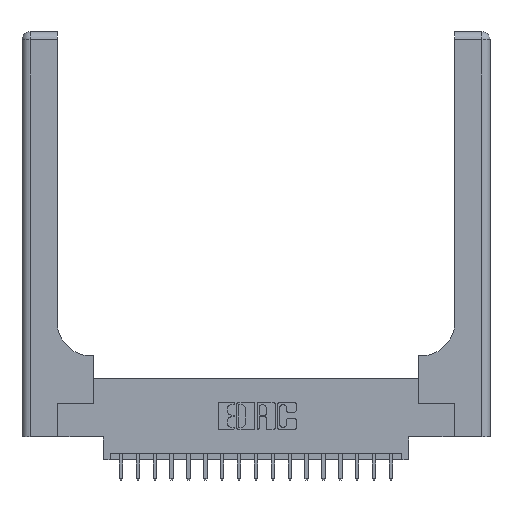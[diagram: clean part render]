
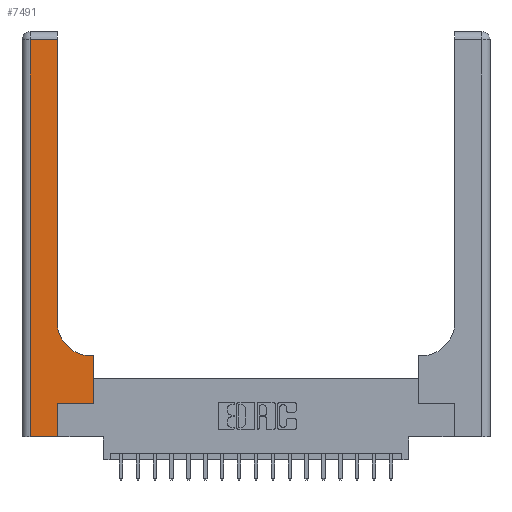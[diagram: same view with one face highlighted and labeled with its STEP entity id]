
A CAD part, top view. The second image highlights one B-rep face of the part: STEP entity #7491.
In plain terms, the highlighted planar face has unit normal (0, 0, 1).
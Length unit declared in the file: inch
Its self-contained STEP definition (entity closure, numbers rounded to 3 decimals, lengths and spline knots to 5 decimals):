
#865 = ORIENTED_EDGE ( 'NONE', *, *, #10429, .T. ) ;
#1348 = EDGE_CURVE ( 'NONE', #14793, #5308, #19549, .T. ) ;
#1537 = CARTESIAN_POINT ( 'NONE',  ( 0.265, 0.25, 0.37 ) ) ;
#1739 = VECTOR ( 'NONE', #1818, 39.37008 ) ;
#1818 = DIRECTION ( 'NONE',  ( 0., -1., 0. ) ) ;
#1980 = DIRECTION ( 'NONE',  ( 0., 1., 0. ) ) ;
#2242 = LINE ( 'NONE', #11277, #1739 ) ;
#2563 = CIRCLE ( 'NONE', #2577, 0.25 ) ;
#2577 = AXIS2_PLACEMENT_3D ( 'NONE', #15284, #6042, #16761 ) ;
#2864 = VERTEX_POINT ( 'NONE', #17548 ) ;
#2959 = CARTESIAN_POINT ( 'NONE',  ( 0., 3., 0.37 ) ) ;
#3204 = DIRECTION ( 'NONE',  ( 0., 1., 0. ) ) ;
#3697 = VERTEX_POINT ( 'NONE', #8237 ) ;
#4343 = CARTESIAN_POINT ( 'NONE',  ( 0.06, 0., 0.37 ) ) ;
#4528 = PLANE ( 'NONE',  #14381 ) ;
#4826 = CARTESIAN_POINT ( 'NONE',  ( 0.265, 0.25, 0.37 ) ) ;
#4950 = EDGE_CURVE ( 'NONE', #11500, #2864, #13025, .T. ) ;
#5244 = VECTOR ( 'NONE', #3204, 39.37008 ) ;
#5308 = VERTEX_POINT ( 'NONE', #11873 ) ;
#5364 = VECTOR ( 'NONE', #16694, 39.37008 ) ;
#5573 = ORIENTED_EDGE ( 'NONE', *, *, #7955, .T. ) ;
#6042 = DIRECTION ( 'NONE',  ( 0., 0., -1. ) ) ;
#6117 = ORIENTED_EDGE ( 'NONE', *, *, #15501, .T. ) ;
#6447 = DIRECTION ( 'NONE',  ( 1., 0., 0. ) ) ;
#7491 = ADVANCED_FACE ( 'NONE', ( #10325 ), #4528, .F. ) ;
#7574 = CARTESIAN_POINT ( 'NONE',  ( 0.26, 0.6, 0.37 ) ) ;
#7740 = DIRECTION ( 'NONE',  ( 0., 0., -1. ) ) ;
#7759 = CARTESIAN_POINT ( 'NONE',  ( 0.26, 0.85, 0.37 ) ) ;
#7955 = EDGE_CURVE ( 'NONE', #2864, #19675, #14845, .T. ) ;
#7995 = VERTEX_POINT ( 'NONE', #8949 ) ;
#8088 = VECTOR ( 'NONE', #19227, 39.37008 ) ;
#8237 = CARTESIAN_POINT ( 'NONE',  ( 0.51, 0.6, 0.37 ) ) ;
#8383 = EDGE_CURVE ( 'NONE', #5308, #17710, #15732, .T. ) ;
#8949 = CARTESIAN_POINT ( 'NONE',  ( 0.528, 0.6, 0.37 ) ) ;
#9276 = ORIENTED_EDGE ( 'NONE', *, *, #4950, .T. ) ;
#9559 = LINE ( 'NONE', #7574, #5364 ) ;
#9613 = ORIENTED_EDGE ( 'NONE', *, *, #1348, .T. ) ;
#10207 = LINE ( 'NONE', #10855, #14757 ) ;
#10325 = FACE_OUTER_BOUND ( 'NONE', #14860, .T. ) ;
#10360 = ORIENTED_EDGE ( 'NONE', *, *, #17113, .T. ) ;
#10429 = EDGE_CURVE ( 'NONE', #14585, #7995, #10207, .T. ) ;
#10855 = CARTESIAN_POINT ( 'NONE',  ( 0.528, 0.25, 0.37 ) ) ;
#11277 = CARTESIAN_POINT ( 'NONE',  ( 0.06, 3., 0.37 ) ) ;
#11500 = VERTEX_POINT ( 'NONE', #7759 ) ;
#11726 = VECTOR ( 'NONE', #1980, 39.37008 ) ;
#11750 = CARTESIAN_POINT ( 'NONE',  ( 0.528, 0.25, 0.37 ) ) ;
#11873 = CARTESIAN_POINT ( 'NONE',  ( 0.265, 0., 0.37 ) ) ;
#11897 = CARTESIAN_POINT ( 'NONE',  ( 0., 2.94, 0.37 ) ) ;
#13025 = LINE ( 'NONE', #14097, #5244 ) ;
#13039 = ORIENTED_EDGE ( 'NONE', *, *, #14248, .T. ) ;
#13261 = ORIENTED_EDGE ( 'NONE', *, *, #8383, .T. ) ;
#14097 = CARTESIAN_POINT ( 'NONE',  ( 0.26, 3., 0.37 ) ) ;
#14248 = EDGE_CURVE ( 'NONE', #3697, #11500, #2563, .T. ) ;
#14381 = AXIS2_PLACEMENT_3D ( 'NONE', #2959, #7740, #18306 ) ;
#14585 = VERTEX_POINT ( 'NONE', #11750 ) ;
#14757 = VECTOR ( 'NONE', #18292, 39.37008 ) ;
#14793 = VERTEX_POINT ( 'NONE', #4343 ) ;
#14845 = LINE ( 'NONE', #11897, #18707 ) ;
#14860 = EDGE_LOOP ( 'NONE', ( #9276, #5573, #6117, #9613, #13261, #10360, #865, #16363, #13039 ) ) ;
#14968 = DIRECTION ( 'NONE',  ( -1., 0., 0. ) ) ;
#15284 = CARTESIAN_POINT ( 'NONE',  ( 0.51, 0.85, 0.37 ) ) ;
#15501 = EDGE_CURVE ( 'NONE', #19675, #14793, #2242, .T. ) ;
#15732 = LINE ( 'NONE', #17381, #11726 ) ;
#16363 = ORIENTED_EDGE ( 'NONE', *, *, #17878, .T. ) ;
#16694 = DIRECTION ( 'NONE',  ( -1., 0., 0. ) ) ;
#16757 = CARTESIAN_POINT ( 'NONE',  ( 0.06, 2.94, 0.37 ) ) ;
#16761 = DIRECTION ( 'NONE',  ( 1., 0., 0. ) ) ;
#17113 = EDGE_CURVE ( 'NONE', #17710, #14585, #18730, .T. ) ;
#17381 = CARTESIAN_POINT ( 'NONE',  ( 0.265, 0., 0.37 ) ) ;
#17548 = CARTESIAN_POINT ( 'NONE',  ( 0.26, 2.94, 0.37 ) ) ;
#17710 = VERTEX_POINT ( 'NONE', #1537 ) ;
#17878 = EDGE_CURVE ( 'NONE', #7995, #3697, #9559, .T. ) ;
#18292 = DIRECTION ( 'NONE',  ( 0., 1., 0. ) ) ;
#18306 = DIRECTION ( 'NONE',  ( -1., 0., 0. ) ) ;
#18707 = VECTOR ( 'NONE', #14968, 39.37008 ) ;
#18730 = LINE ( 'NONE', #4826, #19179 ) ;
#19179 = VECTOR ( 'NONE', #6447, 39.37008 ) ;
#19202 = CARTESIAN_POINT ( 'NONE',  ( 0., 0., 0.37 ) ) ;
#19227 = DIRECTION ( 'NONE',  ( 1., 0., 0. ) ) ;
#19549 = LINE ( 'NONE', #19202, #8088 ) ;
#19675 = VERTEX_POINT ( 'NONE', #16757 ) ;
